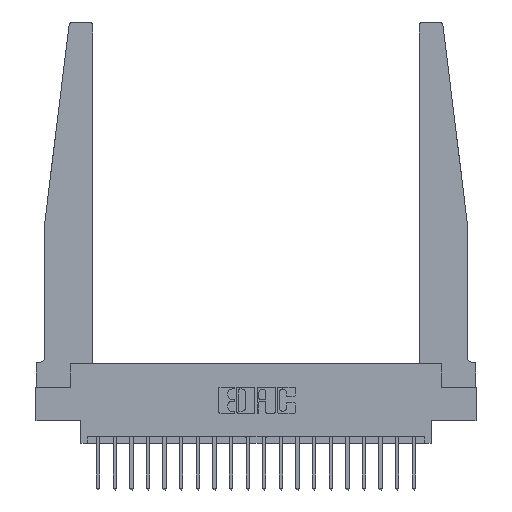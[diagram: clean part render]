
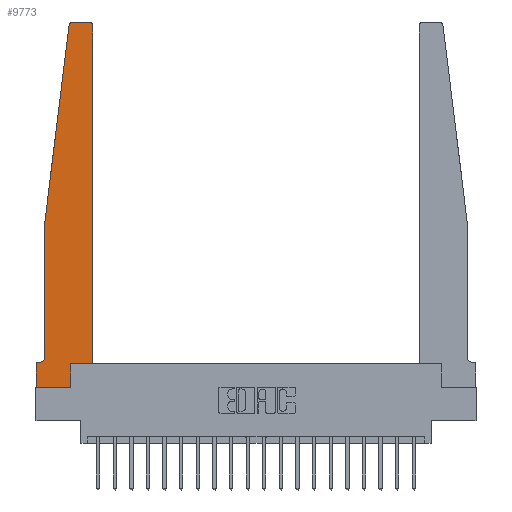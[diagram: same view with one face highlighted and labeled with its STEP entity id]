
A CAD part, top view. The second image highlights one B-rep face of the part: STEP entity #9773.
In plain terms, the highlighted planar face has unit normal (0, 0, 1).
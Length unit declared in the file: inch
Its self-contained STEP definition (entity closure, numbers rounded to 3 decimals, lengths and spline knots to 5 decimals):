
#106 = VECTOR ( 'NONE', #16795, 39.37008 ) ;
#179 = VERTEX_POINT ( 'NONE', #7168 ) ;
#298 = VERTEX_POINT ( 'NONE', #19568 ) ;
#519 = VECTOR ( 'NONE', #10494, 39.37008 ) ;
#1436 = CARTESIAN_POINT ( 'NONE',  ( 0.065, 1.25, 0.37 ) ) ;
#1556 = DIRECTION ( 'NONE',  ( 0., 0., 1. ) ) ;
#1572 = CARTESIAN_POINT ( 'NONE',  ( 0.25, 2.75, 0.37 ) ) ;
#1653 = DIRECTION ( 'NONE',  ( 0., -1., 0. ) ) ;
#1656 = DIRECTION ( 'NONE',  ( 1., 0., 0. ) ) ;
#1941 = LINE ( 'NONE', #6718, #10607 ) ;
#1990 = ORIENTED_EDGE ( 'NONE', *, *, #9828, .T. ) ;
#2133 = ORIENTED_EDGE ( 'NONE', *, *, #15140, .T. ) ;
#2304 = EDGE_CURVE ( 'NONE', #9460, #3539, #21326, .T. ) ;
#2753 = DIRECTION ( 'NONE',  ( -1., 0., 0. ) ) ;
#2861 = DIRECTION ( 'NONE',  ( 0., 0., -1. ) ) ;
#3301 = ORIENTED_EDGE ( 'NONE', *, *, #13495, .T. ) ;
#3457 = CARTESIAN_POINT ( 'NONE',  ( 0., 0., 0.37 ) ) ;
#3539 = VERTEX_POINT ( 'NONE', #15961 ) ;
#3810 = CARTESIAN_POINT ( 'NONE',  ( 0.425, 0.18, 0.37 ) ) ;
#4274 = CARTESIAN_POINT ( 'NONE',  ( 0.2605, 0.18, 0.37 ) ) ;
#4496 = CARTESIAN_POINT ( 'NONE',  ( 0.015, 0.2375, 0.37 ) ) ;
#4519 = CIRCLE ( 'NONE', #20052, 0.05 ) ;
#4770 = PLANE ( 'NONE',  #19885 ) ;
#4886 = ORIENTED_EDGE ( 'NONE', *, *, #15248, .T. ) ;
#4909 = ORIENTED_EDGE ( 'NONE', *, *, #17121, .T. ) ;
#4924 = VERTEX_POINT ( 'NONE', #19374 ) ;
#4982 = ORIENTED_EDGE ( 'NONE', *, *, #2304, .T. ) ;
#5000 = LINE ( 'NONE', #18253, #18407 ) ;
#5852 = VERTEX_POINT ( 'NONE', #6911 ) ;
#5959 = CARTESIAN_POINT ( 'NONE',  ( 0.425, 0.18, 0.37 ) ) ;
#6145 = VERTEX_POINT ( 'NONE', #16180 ) ;
#6182 = FACE_OUTER_BOUND ( 'NONE', #10544, .T. ) ;
#6438 = CARTESIAN_POINT ( 'NONE',  ( 0.27653, 2.72, 0.37 ) ) ;
#6504 = ORIENTED_EDGE ( 'NONE', *, *, #15820, .T. ) ;
#6718 = CARTESIAN_POINT ( 'NONE',  ( 0.065, 0.1875, 0.37 ) ) ;
#6911 = CARTESIAN_POINT ( 'NONE',  ( 0.425, 0.18, 0.37 ) ) ;
#7168 = CARTESIAN_POINT ( 'NONE',  ( 0.015, 0.1875, 0.37 ) ) ;
#7898 = DIRECTION ( 'NONE',  ( 0., 0., 1. ) ) ;
#8546 = DIRECTION ( 'NONE',  ( -1., 0., 0. ) ) ;
#8645 = ORIENTED_EDGE ( 'NONE', *, *, #12425, .T. ) ;
#8949 = VERTEX_POINT ( 'NONE', #18003 ) ;
#8990 = CARTESIAN_POINT ( 'NONE',  ( 0.425, 2.72, 0.37 ) ) ;
#9184 = CARTESIAN_POINT ( 'NONE',  ( 0.24675, 2.72367, 0.37 ) ) ;
#9412 = DIRECTION ( 'NONE',  ( 1., 0., 0. ) ) ;
#9460 = VERTEX_POINT ( 'NONE', #8990 ) ;
#9580 = EDGE_CURVE ( 'NONE', #5852, #9460, #14154, .T. ) ;
#9773 = ADVANCED_FACE ( 'NONE', ( #6182 ), #4770, .T. ) ;
#9828 = EDGE_CURVE ( 'NONE', #179, #6145, #1941, .T. ) ;
#9881 = CARTESIAN_POINT ( 'NONE',  ( 0.395, 2.72, 0.37 ) ) ;
#10130 = ORIENTED_EDGE ( 'NONE', *, *, #10381, .T. ) ;
#10366 = LINE ( 'NONE', #3457, #10815 ) ;
#10381 = EDGE_CURVE ( 'NONE', #8949, #298, #17345, .T. ) ;
#10494 = DIRECTION ( 'NONE',  ( 0., 1., 0. ) ) ;
#10544 = EDGE_LOOP ( 'NONE', ( #3301, #13562, #6504, #2133, #16823, #1990, #4909, #8645, #10130, #4886, #11557, #4982 ) ) ;
#10607 = VECTOR ( 'NONE', #8546, 39.37008 ) ;
#10815 = VECTOR ( 'NONE', #16864, 39.37008 ) ;
#11020 = CARTESIAN_POINT ( 'NONE',  ( 0., 0.1875, 0.37 ) ) ;
#11094 = VECTOR ( 'NONE', #17883, 39.37008 ) ;
#11557 = ORIENTED_EDGE ( 'NONE', *, *, #9580, .T. ) ;
#12304 = CIRCLE ( 'NONE', #17144, 0.03 ) ;
#12362 = EDGE_CURVE ( 'NONE', #18991, #179, #4519, .T. ) ;
#12409 = VECTOR ( 'NONE', #20922, 39.37008 ) ;
#12425 = EDGE_CURVE ( 'NONE', #4924, #8949, #16057, .T. ) ;
#13495 = EDGE_CURVE ( 'NONE', #3539, #16808, #19294, .T. ) ;
#13562 = ORIENTED_EDGE ( 'NONE', *, *, #20559, .T. ) ;
#13717 = AXIS2_PLACEMENT_3D ( 'NONE', #9881, #1556, #18194 ) ;
#14154 = LINE ( 'NONE', #5959, #519 ) ;
#14532 = DIRECTION ( 'NONE',  ( 1., 0., 0. ) ) ;
#15140 = EDGE_CURVE ( 'NONE', #17010, #18991, #16036, .T. ) ;
#15163 = LINE ( 'NONE', #3810, #106 ) ;
#15248 = EDGE_CURVE ( 'NONE', #298, #5852, #15163, .T. ) ;
#15820 = EDGE_CURVE ( 'NONE', #18669, #17010, #5000, .T. ) ;
#15841 = CARTESIAN_POINT ( 'NONE',  ( 0.065, 0.2375, 0.37 ) ) ;
#15961 = CARTESIAN_POINT ( 'NONE',  ( 0.395, 2.75, 0.37 ) ) ;
#16036 = LINE ( 'NONE', #1436, #17357 ) ;
#16057 = LINE ( 'NONE', #19908, #17620 ) ;
#16180 = CARTESIAN_POINT ( 'NONE',  ( 0., 0.1875, 0.37 ) ) ;
#16654 = DIRECTION ( 'NONE',  ( -0.122, -0.992, 0. ) ) ;
#16795 = DIRECTION ( 'NONE',  ( 1., 0., 0. ) ) ;
#16808 = VERTEX_POINT ( 'NONE', #17291 ) ;
#16823 = ORIENTED_EDGE ( 'NONE', *, *, #12362, .T. ) ;
#16864 = DIRECTION ( 'NONE',  ( 0., -1., 0. ) ) ;
#17010 = VERTEX_POINT ( 'NONE', #19774 ) ;
#17121 = EDGE_CURVE ( 'NONE', #6145, #4924, #10366, .T. ) ;
#17144 = AXIS2_PLACEMENT_3D ( 'NONE', #6438, #18081, #1656 ) ;
#17291 = CARTESIAN_POINT ( 'NONE',  ( 0.27653, 2.75, 0.37 ) ) ;
#17345 = LINE ( 'NONE', #4274, #12409 ) ;
#17357 = VECTOR ( 'NONE', #1653, 39.37008 ) ;
#17620 = VECTOR ( 'NONE', #14532, 39.37008 ) ;
#17883 = DIRECTION ( 'NONE',  ( -1., 0., 0. ) ) ;
#18003 = CARTESIAN_POINT ( 'NONE',  ( 0.2605, 0., 0.37 ) ) ;
#18081 = DIRECTION ( 'NONE',  ( 0., 0., 1. ) ) ;
#18194 = DIRECTION ( 'NONE',  ( 1., 0., 0. ) ) ;
#18253 = CARTESIAN_POINT ( 'NONE',  ( 0.065, 1.25, 0.37 ) ) ;
#18407 = VECTOR ( 'NONE', #16654, 39.37008 ) ;
#18669 = VERTEX_POINT ( 'NONE', #9184 ) ;
#18991 = VERTEX_POINT ( 'NONE', #15841 ) ;
#19294 = LINE ( 'NONE', #1572, #11094 ) ;
#19374 = CARTESIAN_POINT ( 'NONE',  ( 0., 0., 0.37 ) ) ;
#19568 = CARTESIAN_POINT ( 'NONE',  ( 0.2605, 0.18, 0.37 ) ) ;
#19774 = CARTESIAN_POINT ( 'NONE',  ( 0.065, 1.25, 0.37 ) ) ;
#19885 = AXIS2_PLACEMENT_3D ( 'NONE', #11020, #7898, #9412 ) ;
#19908 = CARTESIAN_POINT ( 'NONE',  ( 0., 0., 0.37 ) ) ;
#20052 = AXIS2_PLACEMENT_3D ( 'NONE', #4496, #2861, #2753 ) ;
#20559 = EDGE_CURVE ( 'NONE', #16808, #18669, #12304, .T. ) ;
#20922 = DIRECTION ( 'NONE',  ( 0., 1., 0. ) ) ;
#21326 = CIRCLE ( 'NONE', #13717, 0.03 ) ;
